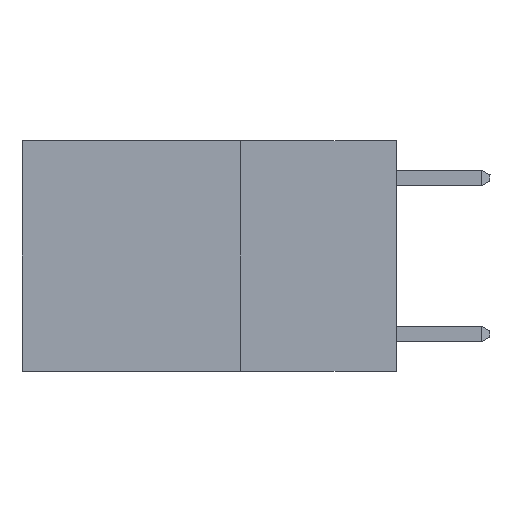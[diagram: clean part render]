
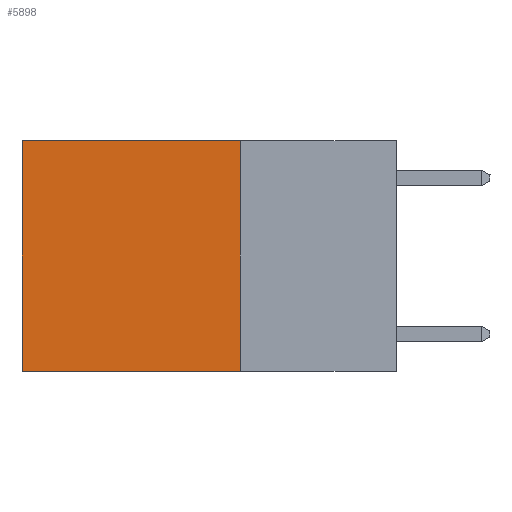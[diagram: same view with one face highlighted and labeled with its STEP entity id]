
A CAD part, left-side view. The second image highlights one B-rep face of the part: STEP entity #5898.
In plain terms, the highlighted planar face has unit normal (-1, 0, 0).
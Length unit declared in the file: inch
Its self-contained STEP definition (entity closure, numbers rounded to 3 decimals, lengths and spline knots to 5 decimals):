
#90 = PLANE ( 'NONE',  #8058 ) ;
#497 = EDGE_LOOP ( 'NONE', ( #7888, #7417, #10678, #8471 ) ) ;
#499 = EDGE_CURVE ( 'NONE', #8837, #2862, #954, .T. ) ;
#680 = DIRECTION ( 'NONE',  ( 0., 1., 0. ) ) ;
#954 = LINE ( 'NONE', #5477, #9454 ) ;
#963 = CARTESIAN_POINT ( 'NONE',  ( 0.2625, 0.25, 0. ) ) ;
#1055 = VERTEX_POINT ( 'NONE', #6793 ) ;
#1368 = VECTOR ( 'NONE', #680, 39.37008 ) ;
#1804 = DIRECTION ( 'NONE',  ( 0., 0., -1. ) ) ;
#1947 = CARTESIAN_POINT ( 'NONE',  ( 0.2625, 0.25, -0.37 ) ) ;
#2692 = EDGE_CURVE ( 'NONE', #1055, #8837, #8445, .T. ) ;
#2862 = VERTEX_POINT ( 'NONE', #8282 ) ;
#3457 = FACE_OUTER_BOUND ( 'NONE', #497, .T. ) ;
#3698 = VERTEX_POINT ( 'NONE', #1947 ) ;
#3802 = DIRECTION ( 'NONE',  ( 0., 1., 0. ) ) ;
#5477 = CARTESIAN_POINT ( 'NONE',  ( 0.2625, 0.6, 0. ) ) ;
#5502 = CARTESIAN_POINT ( 'NONE',  ( 0.2625, 0.25, 0. ) ) ;
#5669 = CARTESIAN_POINT ( 'NONE',  ( 0.2625, 0.25, 0. ) ) ;
#5898 = ADVANCED_FACE ( 'NONE', ( #3457 ), #90, .F. ) ;
#6793 = CARTESIAN_POINT ( 'NONE',  ( 0.2625, 0.25, 0. ) ) ;
#6824 = DIRECTION ( 'NONE',  ( 1., 0., 0. ) ) ;
#7255 = EDGE_CURVE ( 'NONE', #1055, #3698, #7857, .T. ) ;
#7417 = ORIENTED_EDGE ( 'NONE', *, *, #9101, .F. ) ;
#7570 = VECTOR ( 'NONE', #9146, 39.37008 ) ;
#7586 = DIRECTION ( 'NONE',  ( 0., 0., -1. ) ) ;
#7857 = LINE ( 'NONE', #5669, #7570 ) ;
#7888 = ORIENTED_EDGE ( 'NONE', *, *, #499, .T. ) ;
#8058 = AXIS2_PLACEMENT_3D ( 'NONE', #963, #6824, #1804 ) ;
#8282 = CARTESIAN_POINT ( 'NONE',  ( 0.2625, 0.6, -0.37 ) ) ;
#8445 = LINE ( 'NONE', #5502, #10734 ) ;
#8471 = ORIENTED_EDGE ( 'NONE', *, *, #2692, .T. ) ;
#8626 = CARTESIAN_POINT ( 'NONE',  ( 0.2625, 0.6, 0. ) ) ;
#8837 = VERTEX_POINT ( 'NONE', #8626 ) ;
#9101 = EDGE_CURVE ( 'NONE', #3698, #2862, #10666, .T. ) ;
#9146 = DIRECTION ( 'NONE',  ( 0., 0., -1. ) ) ;
#9454 = VECTOR ( 'NONE', #7586, 39.37008 ) ;
#10010 = CARTESIAN_POINT ( 'NONE',  ( 0.2625, 0.25, -0.37 ) ) ;
#10666 = LINE ( 'NONE', #10010, #1368 ) ;
#10678 = ORIENTED_EDGE ( 'NONE', *, *, #7255, .F. ) ;
#10734 = VECTOR ( 'NONE', #3802, 39.37008 ) ;
